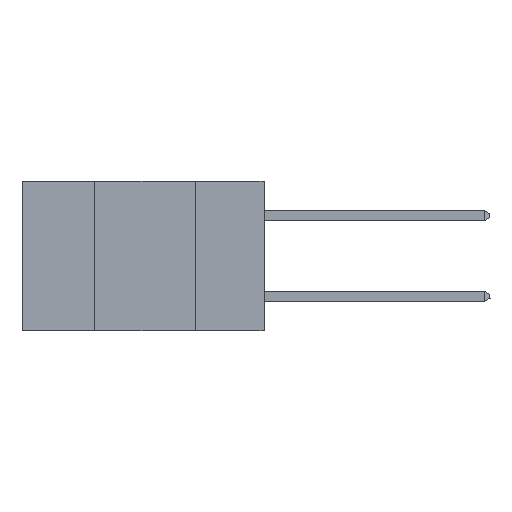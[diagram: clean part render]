
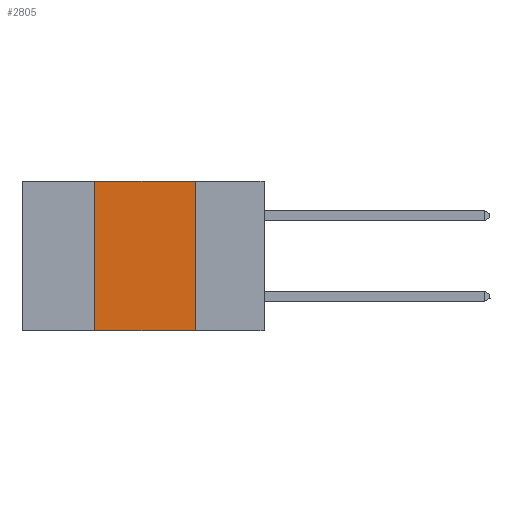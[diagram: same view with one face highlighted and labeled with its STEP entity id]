
A CAD part, left-side view. The second image highlights one B-rep face of the part: STEP entity #2805.
In plain terms, the highlighted planar face has unit normal (-1, 0, 0).
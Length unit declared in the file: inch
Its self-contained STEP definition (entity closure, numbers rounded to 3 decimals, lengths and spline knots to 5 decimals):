
#70 = CARTESIAN_POINT ( 'NONE',  ( 0., 0.6, -0.37 ) ) ;
#205 = ORIENTED_EDGE ( 'NONE', *, *, #7739, .F. ) ;
#669 = CARTESIAN_POINT ( 'NONE',  ( 0., 0.6, 0. ) ) ;
#710 = EDGE_CURVE ( 'NONE', #10216, #8474, #6732, .T. ) ;
#1685 = CARTESIAN_POINT ( 'NONE',  ( 0., 0.17, -0.37 ) ) ;
#1825 = VERTEX_POINT ( 'NONE', #10462 ) ;
#2066 = LINE ( 'NONE', #1685, #7740 ) ;
#2805 = ADVANCED_FACE ( 'NONE', ( #3883 ), #9690, .F. ) ;
#3012 = EDGE_CURVE ( 'NONE', #10216, #1825, #9607, .T. ) ;
#3036 = CARTESIAN_POINT ( 'NONE',  ( 0., 0.17, 0. ) ) ;
#3303 = DIRECTION ( 'NONE',  ( 0., -1., 0. ) ) ;
#3611 = DIRECTION ( 'NONE',  ( 0., -1., 0. ) ) ;
#3883 = FACE_OUTER_BOUND ( 'NONE', #7962, .T. ) ;
#4421 = CARTESIAN_POINT ( 'NONE',  ( 0., 0.42, 0. ) ) ;
#4753 = VERTEX_POINT ( 'NONE', #3036 ) ;
#5050 = DIRECTION ( 'NONE',  ( 1., 0., 0. ) ) ;
#5711 = DIRECTION ( 'NONE',  ( 0., 0., 1. ) ) ;
#6187 = CARTESIAN_POINT ( 'NONE',  ( 0., 0.42, -0.37 ) ) ;
#6732 = LINE ( 'NONE', #7577, #7711 ) ;
#6801 = VECTOR ( 'NONE', #3303, 39.37008 ) ;
#7577 = CARTESIAN_POINT ( 'NONE',  ( 0., 0.42, -0.37 ) ) ;
#7711 = VECTOR ( 'NONE', #5711, 39.37008 ) ;
#7739 = EDGE_CURVE ( 'NONE', #8474, #4753, #10255, .T. ) ;
#7740 = VECTOR ( 'NONE', #8038, 39.37008 ) ;
#7892 = DIRECTION ( 'NONE',  ( 0., 0., -1. ) ) ;
#7962 = EDGE_LOOP ( 'NONE', ( #9034, #205, #10720, #8701 ) ) ;
#8038 = DIRECTION ( 'NONE',  ( 0., 0., -1. ) ) ;
#8473 = VECTOR ( 'NONE', #3611, 39.37008 ) ;
#8474 = VERTEX_POINT ( 'NONE', #4421 ) ;
#8701 = ORIENTED_EDGE ( 'NONE', *, *, #3012, .T. ) ;
#8738 = EDGE_CURVE ( 'NONE', #4753, #1825, #2066, .T. ) ;
#9034 = ORIENTED_EDGE ( 'NONE', *, *, #8738, .F. ) ;
#9607 = LINE ( 'NONE', #70, #8473 ) ;
#9615 = CARTESIAN_POINT ( 'NONE',  ( 0., 0.6, 0. ) ) ;
#9690 = PLANE ( 'NONE',  #10792 ) ;
#10216 = VERTEX_POINT ( 'NONE', #6187 ) ;
#10255 = LINE ( 'NONE', #669, #6801 ) ;
#10462 = CARTESIAN_POINT ( 'NONE',  ( 0., 0.17, -0.37 ) ) ;
#10720 = ORIENTED_EDGE ( 'NONE', *, *, #710, .F. ) ;
#10792 = AXIS2_PLACEMENT_3D ( 'NONE', #9615, #5050, #7892 ) ;
